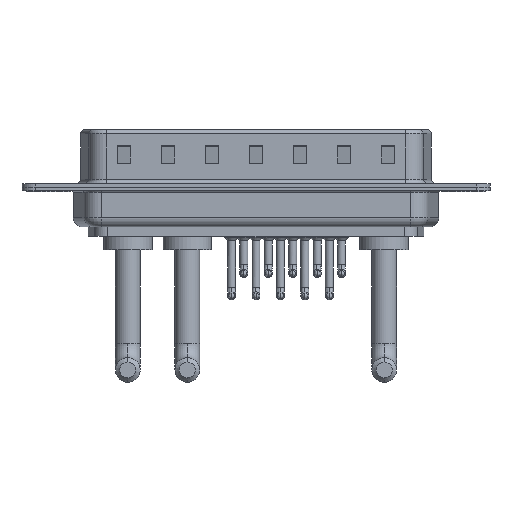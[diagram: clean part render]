
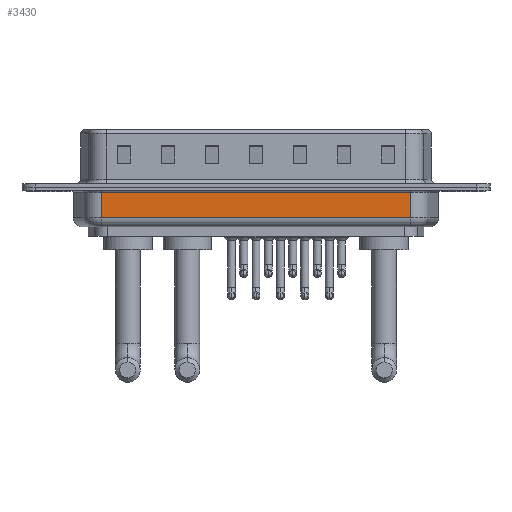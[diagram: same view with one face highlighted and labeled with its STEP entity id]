
A CAD part, front view. The second image highlights one B-rep face of the part: STEP entity #3430.
In plain terms, the highlighted planar face has unit normal (0, -1, 0).
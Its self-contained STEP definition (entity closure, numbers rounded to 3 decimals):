
#291 = DIRECTION ( 'NONE',  ( 0., 0., 1. ) ) ;
#2067 = LINE ( 'NONE', #13639, #7434 ) ;
#2503 = EDGE_CURVE ( 'NONE', #2850, #18958, #3334, .T. ) ;
#2850 = VERTEX_POINT ( 'NONE', #5983 ) ;
#2960 = DIRECTION ( 'NONE',  ( 0., 0., 1. ) ) ;
#3334 = LINE ( 'NONE', #13291, #15470 ) ;
#3430 = ADVANCED_FACE ( 'NONE', ( #6159 ), #4607, .F. ) ;
#3698 = EDGE_CURVE ( 'NONE', #18526, #6209, #2067, .T. ) ;
#4607 = PLANE ( 'NONE',  #16615 ) ;
#4611 = LINE ( 'NONE', #14455, #5343 ) ;
#5024 = CARTESIAN_POINT ( 'NONE',  ( 41.044, -5.35, -4.5 ) ) ;
#5343 = VECTOR ( 'NONE', #2960, 1000. ) ;
#5818 = DIRECTION ( 'NONE',  ( 0., 1., 0. ) ) ;
#5983 = CARTESIAN_POINT ( 'NONE',  ( 6.006, -5.35, -3.5 ) ) ;
#6159 = FACE_OUTER_BOUND ( 'NONE', #19380, .T. ) ;
#6209 = VERTEX_POINT ( 'NONE', #12250 ) ;
#6776 = LINE ( 'NONE', #5024, #21708 ) ;
#7062 = EDGE_CURVE ( 'NONE', #18958, #18526, #6776, .T. ) ;
#7199 = ORIENTED_EDGE ( 'NONE', *, *, #2503, .T. ) ;
#7434 = VECTOR ( 'NONE', #15416, 1000. ) ;
#8917 = EDGE_CURVE ( 'NONE', #2850, #6209, #4611, .T. ) ;
#10450 = CARTESIAN_POINT ( 'NONE',  ( 41.044, -5.35, -0.65 ) ) ;
#10536 = CARTESIAN_POINT ( 'NONE',  ( 41.044, -5.35, -3.5 ) ) ;
#11351 = CARTESIAN_POINT ( 'NONE',  ( 6.006, -5.35, -4.5 ) ) ;
#11869 = ORIENTED_EDGE ( 'NONE', *, *, #8917, .F. ) ;
#12250 = CARTESIAN_POINT ( 'NONE',  ( 6.006, -5.35, -0.65 ) ) ;
#12370 = ORIENTED_EDGE ( 'NONE', *, *, #3698, .T. ) ;
#12977 = DIRECTION ( 'NONE',  ( 1., 0., 0. ) ) ;
#13291 = CARTESIAN_POINT ( 'NONE',  ( 6.006, -5.35, -3.5 ) ) ;
#13639 = CARTESIAN_POINT ( 'NONE',  ( 6.006, -5.35, -0.65 ) ) ;
#13987 = ORIENTED_EDGE ( 'NONE', *, *, #7062, .T. ) ;
#14455 = CARTESIAN_POINT ( 'NONE',  ( 6.006, -5.35, -4.5 ) ) ;
#15416 = DIRECTION ( 'NONE',  ( -1., 0., 0. ) ) ;
#15470 = VECTOR ( 'NONE', #12977, 1000. ) ;
#16615 = AXIS2_PLACEMENT_3D ( 'NONE', #11351, #5818, #18067 ) ;
#18067 = DIRECTION ( 'NONE',  ( 0., 0., 1. ) ) ;
#18526 = VERTEX_POINT ( 'NONE', #10450 ) ;
#18958 = VERTEX_POINT ( 'NONE', #10536 ) ;
#19380 = EDGE_LOOP ( 'NONE', ( #11869, #7199, #13987, #12370 ) ) ;
#21708 = VECTOR ( 'NONE', #291, 1000. ) ;
